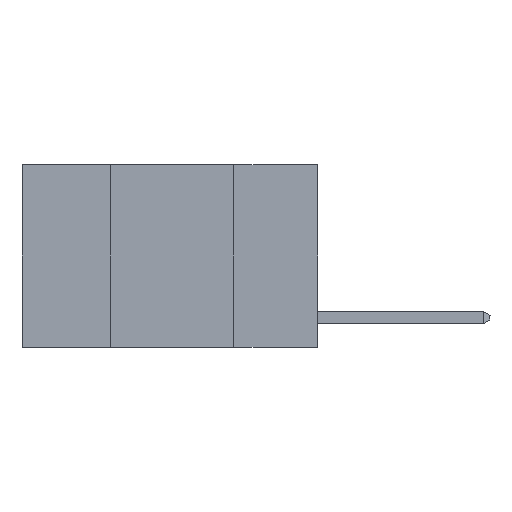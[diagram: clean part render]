
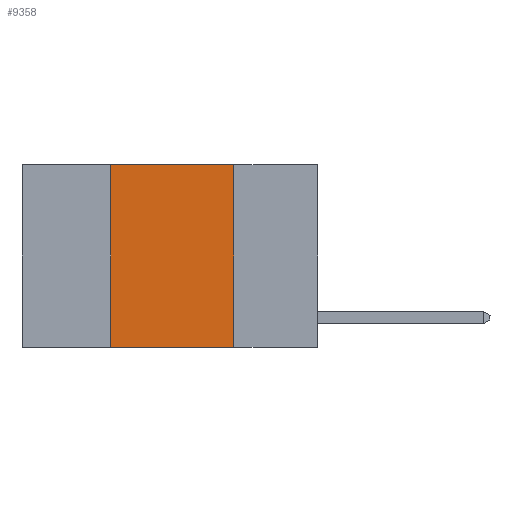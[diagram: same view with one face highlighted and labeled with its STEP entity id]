
A CAD part, left-side view. The second image highlights one B-rep face of the part: STEP entity #9358.
In plain terms, the highlighted planar face has unit normal (-1, 0, 0).
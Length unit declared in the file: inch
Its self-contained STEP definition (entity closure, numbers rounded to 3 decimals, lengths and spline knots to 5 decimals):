
#30 = CARTESIAN_POINT ( 'NONE',  ( 0., 0.17, -0.37 ) ) ;
#894 = DIRECTION ( 'NONE',  ( 1., 0., 0. ) ) ;
#914 = EDGE_CURVE ( 'NONE', #7715, #10299, #1292, .T. ) ;
#1292 = LINE ( 'NONE', #2932, #12270 ) ;
#1424 = CARTESIAN_POINT ( 'NONE',  ( 0., 0.42, -0.37 ) ) ;
#1475 = VECTOR ( 'NONE', #3230, 39.37008 ) ;
#1555 = VERTEX_POINT ( 'NONE', #11077 ) ;
#1598 = EDGE_CURVE ( 'NONE', #7715, #11224, #4284, .T. ) ;
#1600 = EDGE_CURVE ( 'NONE', #1555, #10299, #1764, .T. ) ;
#1764 = LINE ( 'NONE', #6066, #11798 ) ;
#2638 = ORIENTED_EDGE ( 'NONE', *, *, #1600, .F. ) ;
#2932 = CARTESIAN_POINT ( 'NONE',  ( 0., 0.6, -0.37 ) ) ;
#3230 = DIRECTION ( 'NONE',  ( 0., -1., 0. ) ) ;
#3973 = CARTESIAN_POINT ( 'NONE',  ( 0., 0.42, 0. ) ) ;
#4284 = LINE ( 'NONE', #3973, #9468 ) ;
#4909 = AXIS2_PLACEMENT_3D ( 'NONE', #13182, #894, #8243 ) ;
#5036 = DIRECTION ( 'NONE',  ( 0., 0., 1. ) ) ;
#5467 = ORIENTED_EDGE ( 'NONE', *, *, #6914, .F. ) ;
#5794 = ORIENTED_EDGE ( 'NONE', *, *, #914, .T. ) ;
#6066 = CARTESIAN_POINT ( 'NONE',  ( 0., 0.17, 0. ) ) ;
#6823 = EDGE_LOOP ( 'NONE', ( #2638, #5467, #8184, #5794 ) ) ;
#6914 = EDGE_CURVE ( 'NONE', #11224, #1555, #9509, .T. ) ;
#7135 = DIRECTION ( 'NONE',  ( 0., 0., -1. ) ) ;
#7216 = PLANE ( 'NONE',  #4909 ) ;
#7715 = VERTEX_POINT ( 'NONE', #1424 ) ;
#8184 = ORIENTED_EDGE ( 'NONE', *, *, #1598, .F. ) ;
#8243 = DIRECTION ( 'NONE',  ( 0., 0., -1. ) ) ;
#8449 = CARTESIAN_POINT ( 'NONE',  ( 0., 0.6, 0. ) ) ;
#9358 = ADVANCED_FACE ( 'NONE', ( #9911 ), #7216, .F. ) ;
#9468 = VECTOR ( 'NONE', #5036, 39.37008 ) ;
#9509 = LINE ( 'NONE', #8449, #1475 ) ;
#9516 = CARTESIAN_POINT ( 'NONE',  ( 0., 0.42, 0. ) ) ;
#9911 = FACE_OUTER_BOUND ( 'NONE', #6823, .T. ) ;
#10191 = DIRECTION ( 'NONE',  ( 0., -1., 0. ) ) ;
#10299 = VERTEX_POINT ( 'NONE', #30 ) ;
#11077 = CARTESIAN_POINT ( 'NONE',  ( 0., 0.17, 0. ) ) ;
#11224 = VERTEX_POINT ( 'NONE', #9516 ) ;
#11798 = VECTOR ( 'NONE', #7135, 39.37008 ) ;
#12270 = VECTOR ( 'NONE', #10191, 39.37008 ) ;
#13182 = CARTESIAN_POINT ( 'NONE',  ( 0., 0.6, 0. ) ) ;
